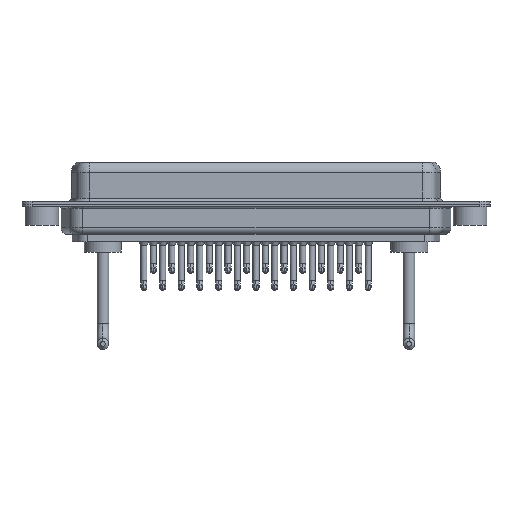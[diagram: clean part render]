
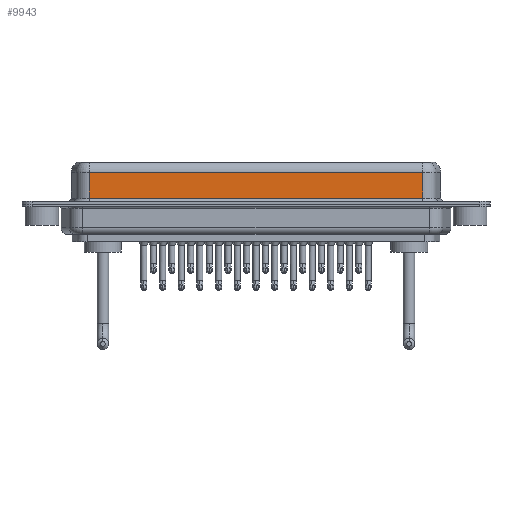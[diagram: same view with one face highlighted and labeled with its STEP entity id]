
A CAD part, front view. The second image highlights one B-rep face of the part: STEP entity #9943.
In plain terms, the highlighted planar face has unit normal (0, -1, 0).
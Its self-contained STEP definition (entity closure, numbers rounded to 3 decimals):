
#418 = DIRECTION ( 'NONE',  ( 0., 0., 1. ) ) ;
#937 = LINE ( 'NONE', #14904, #21713 ) ;
#2019 = VECTOR ( 'NONE', #15593, 1000. ) ;
#2306 = DIRECTION ( 'NONE',  ( 0., 1., 0. ) ) ;
#2616 = VERTEX_POINT ( 'NONE', #22245 ) ;
#2978 = ORIENTED_EDGE ( 'NONE', *, *, #7310, .F. ) ;
#3273 = VERTEX_POINT ( 'NONE', #21800 ) ;
#3460 = LINE ( 'NONE', #13293, #20022 ) ;
#3532 = EDGE_CURVE ( 'NONE', #2616, #3273, #3460, .T. ) ;
#5470 = VERTEX_POINT ( 'NONE', #19708 ) ;
#6144 = CARTESIAN_POINT ( 'NONE',  ( 7.038, -3.95, 6.4 ) ) ;
#7054 = CARTESIAN_POINT ( 'NONE',  ( 56.462, -3.95, 0.9 ) ) ;
#7173 = DIRECTION ( 'NONE',  ( 1., 0., 0. ) ) ;
#7310 = EDGE_CURVE ( 'NONE', #2616, #5470, #937, .T. ) ;
#7853 = FACE_OUTER_BOUND ( 'NONE', #13507, .T. ) ;
#8484 = ORIENTED_EDGE ( 'NONE', *, *, #3532, .T. ) ;
#9048 = CARTESIAN_POINT ( 'NONE',  ( 7.038, -3.95, 0.9 ) ) ;
#9148 = DIRECTION ( 'NONE',  ( -1., 0., 0. ) ) ;
#9943 = ADVANCED_FACE ( 'NONE', ( #7853 ), #13771, .F. ) ;
#10464 = ORIENTED_EDGE ( 'NONE', *, *, #10874, .T. ) ;
#10874 = EDGE_CURVE ( 'NONE', #3273, #19849, #21237, .T. ) ;
#12049 = VECTOR ( 'NONE', #7173, 1000. ) ;
#13293 = CARTESIAN_POINT ( 'NONE',  ( 56.462, -3.95, 4.65 ) ) ;
#13507 = EDGE_LOOP ( 'NONE', ( #2978, #8484, #10464, #17832 ) ) ;
#13771 = PLANE ( 'NONE',  #13822 ) ;
#13822 = AXIS2_PLACEMENT_3D ( 'NONE', #19538, #2306, #418 ) ;
#14904 = CARTESIAN_POINT ( 'NONE',  ( 56.462, -3.95, 6.4 ) ) ;
#15593 = DIRECTION ( 'NONE',  ( 0., 0., -1. ) ) ;
#16290 = DIRECTION ( 'NONE',  ( 0., 0., -1. ) ) ;
#17832 = ORIENTED_EDGE ( 'NONE', *, *, #23819, .T. ) ;
#19538 = CARTESIAN_POINT ( 'NONE',  ( 56.462, -3.95, 6.4 ) ) ;
#19708 = CARTESIAN_POINT ( 'NONE',  ( 56.462, -3.95, 0.9 ) ) ;
#19849 = VERTEX_POINT ( 'NONE', #9048 ) ;
#20022 = VECTOR ( 'NONE', #9148, 1000. ) ;
#20769 = LINE ( 'NONE', #7054, #12049 ) ;
#21237 = LINE ( 'NONE', #6144, #2019 ) ;
#21713 = VECTOR ( 'NONE', #16290, 1000. ) ;
#21800 = CARTESIAN_POINT ( 'NONE',  ( 7.038, -3.95, 4.65 ) ) ;
#22245 = CARTESIAN_POINT ( 'NONE',  ( 56.462, -3.95, 4.65 ) ) ;
#23819 = EDGE_CURVE ( 'NONE', #19849, #5470, #20769, .T. ) ;
